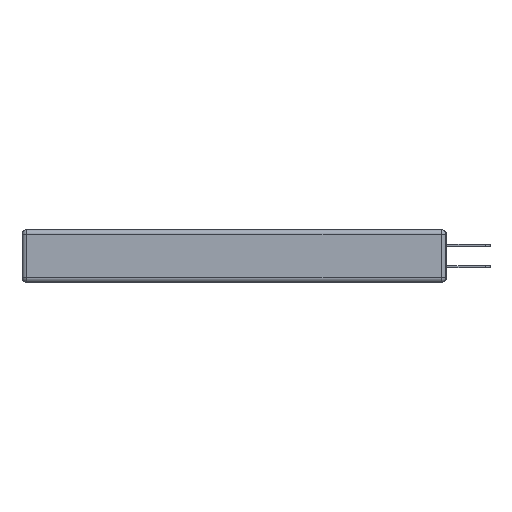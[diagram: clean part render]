
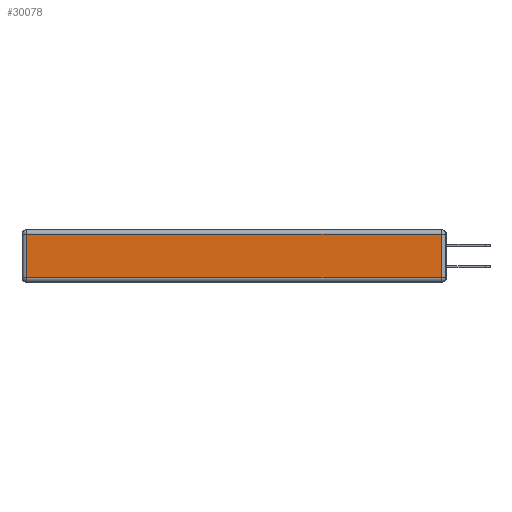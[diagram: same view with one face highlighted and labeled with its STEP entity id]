
A CAD part, left-side view. The second image highlights one B-rep face of the part: STEP entity #30078.
In plain terms, the highlighted planar face has unit normal (-1, 0, 0).
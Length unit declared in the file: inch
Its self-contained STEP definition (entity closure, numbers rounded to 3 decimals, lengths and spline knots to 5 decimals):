
#112 = LINE ( 'NONE', #4529, #3000 ) ;
#150 = EDGE_CURVE ( 'NONE', #20588, #14872, #33719, .T. ) ;
#1794 = LINE ( 'NONE', #10823, #28694 ) ;
#3000 = VECTOR ( 'NONE', #4642, 39.37008 ) ;
#4529 = CARTESIAN_POINT ( 'NONE',  ( 0., 0., -0.313 ) ) ;
#4642 = DIRECTION ( 'NONE',  ( 0., -1., 0. ) ) ;
#5493 = VECTOR ( 'NONE', #30657, 39.37008 ) ;
#6253 = EDGE_CURVE ( 'NONE', #15733, #20588, #1794, .T. ) ;
#6356 = LINE ( 'NONE', #32936, #5493 ) ;
#6629 = DIRECTION ( 'NONE',  ( -1., 0., 0. ) ) ;
#6690 = CARTESIAN_POINT ( 'NONE',  ( 0., 0.03, -0.313 ) ) ;
#7745 = EDGE_LOOP ( 'NONE', ( #22431, #19961, #33449, #18035 ) ) ;
#9200 = DIRECTION ( 'NONE',  ( 0., 0., 1. ) ) ;
#10508 = DIRECTION ( 'NONE',  ( 0., 0., -1. ) ) ;
#10823 = CARTESIAN_POINT ( 'NONE',  ( 0., 2.75, -0.03 ) ) ;
#13995 = VERTEX_POINT ( 'NONE', #6690 ) ;
#14311 = CARTESIAN_POINT ( 'NONE',  ( 0., 0.03, -0.03 ) ) ;
#14872 = VERTEX_POINT ( 'NONE', #16524 ) ;
#15655 = CARTESIAN_POINT ( 'NONE',  ( 0., 2.72, -0.343 ) ) ;
#15733 = VERTEX_POINT ( 'NONE', #14311 ) ;
#16355 = AXIS2_PLACEMENT_3D ( 'NONE', #24732, #6629, #9200 ) ;
#16513 = EDGE_CURVE ( 'NONE', #13995, #15733, #6356, .T. ) ;
#16524 = CARTESIAN_POINT ( 'NONE',  ( 0., 2.72, -0.313 ) ) ;
#18035 = ORIENTED_EDGE ( 'NONE', *, *, #150, .T. ) ;
#18241 = EDGE_CURVE ( 'NONE', #14872, #13995, #112, .T. ) ;
#19605 = CARTESIAN_POINT ( 'NONE',  ( 0., 2.72, -0.03 ) ) ;
#19961 = ORIENTED_EDGE ( 'NONE', *, *, #16513, .T. ) ;
#20588 = VERTEX_POINT ( 'NONE', #19605 ) ;
#22431 = ORIENTED_EDGE ( 'NONE', *, *, #18241, .T. ) ;
#24732 = CARTESIAN_POINT ( 'NONE',  ( 0., 0., -0.343 ) ) ;
#27585 = PLANE ( 'NONE',  #16355 ) ;
#28001 = VECTOR ( 'NONE', #10508, 39.37008 ) ;
#28694 = VECTOR ( 'NONE', #29443, 39.37008 ) ;
#29443 = DIRECTION ( 'NONE',  ( 0., 1., 0. ) ) ;
#30078 = ADVANCED_FACE ( 'NONE', ( #32104 ), #27585, .T. ) ;
#30657 = DIRECTION ( 'NONE',  ( 0., 0., 1. ) ) ;
#32104 = FACE_OUTER_BOUND ( 'NONE', #7745, .T. ) ;
#32936 = CARTESIAN_POINT ( 'NONE',  ( 0., 0.03, -0.343 ) ) ;
#33449 = ORIENTED_EDGE ( 'NONE', *, *, #6253, .T. ) ;
#33719 = LINE ( 'NONE', #15655, #28001 ) ;
